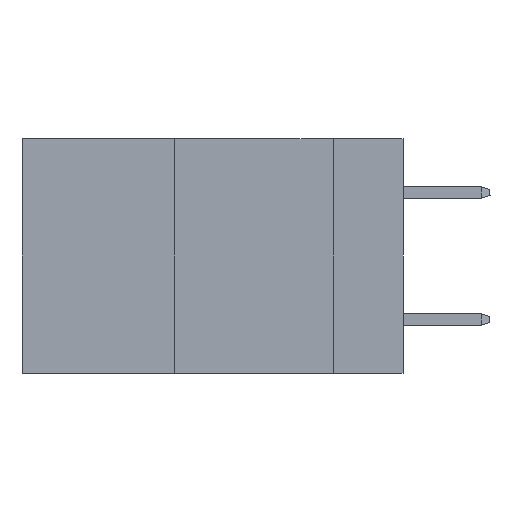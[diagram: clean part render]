
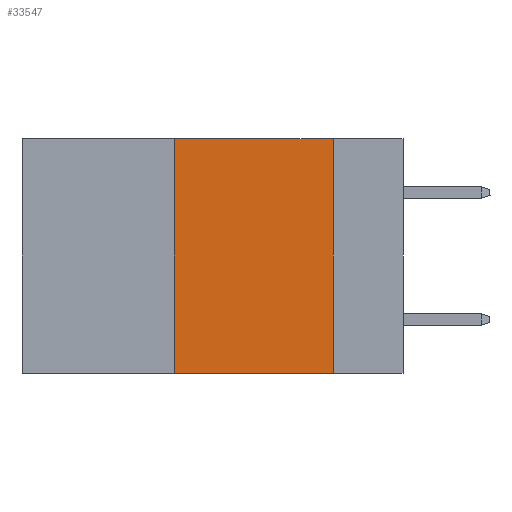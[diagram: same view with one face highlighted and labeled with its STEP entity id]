
A CAD part, left-side view. The second image highlights one B-rep face of the part: STEP entity #33547.
In plain terms, the highlighted planar face has unit normal (-1, 0, 0).
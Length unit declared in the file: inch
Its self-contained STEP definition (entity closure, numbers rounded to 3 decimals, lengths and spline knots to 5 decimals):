
#686 = VECTOR ( 'NONE', #26114, 39.37008 ) ;
#1525 = VERTEX_POINT ( 'NONE', #5872 ) ;
#2205 = EDGE_CURVE ( 'NONE', #9310, #1525, #44298, .T. ) ;
#3482 = DIRECTION ( 'NONE',  ( 0., -1., 0. ) ) ;
#5020 = ORIENTED_EDGE ( 'NONE', *, *, #42511, .F. ) ;
#5127 = EDGE_LOOP ( 'NONE', ( #23720, #5020, #41222, #33146 ) ) ;
#5872 = CARTESIAN_POINT ( 'NONE',  ( 0., 0.11, -0.37 ) ) ;
#6529 = VERTEX_POINT ( 'NONE', #11088 ) ;
#9310 = VERTEX_POINT ( 'NONE', #23360 ) ;
#9339 = LINE ( 'NONE', #17311, #20609 ) ;
#10568 = VERTEX_POINT ( 'NONE', #29339 ) ;
#11088 = CARTESIAN_POINT ( 'NONE',  ( 0., 0.36, 0. ) ) ;
#13699 = VECTOR ( 'NONE', #40795, 39.37008 ) ;
#15322 = EDGE_CURVE ( 'NONE', #10568, #6529, #9339, .T. ) ;
#17311 = CARTESIAN_POINT ( 'NONE',  ( 0., 0.36, 0. ) ) ;
#19581 = AXIS2_PLACEMENT_3D ( 'NONE', #23146, #37807, #26535 ) ;
#20609 = VECTOR ( 'NONE', #24756, 39.37008 ) ;
#22548 = CARTESIAN_POINT ( 'NONE',  ( 0., 0.6, -0.37 ) ) ;
#22710 = CARTESIAN_POINT ( 'NONE',  ( 0., 0.11, 0. ) ) ;
#23146 = CARTESIAN_POINT ( 'NONE',  ( 0., 0.6, 0. ) ) ;
#23360 = CARTESIAN_POINT ( 'NONE',  ( 0., 0.11, 0. ) ) ;
#23720 = ORIENTED_EDGE ( 'NONE', *, *, #2205, .F. ) ;
#24756 = DIRECTION ( 'NONE',  ( 0., 0., 1. ) ) ;
#26114 = DIRECTION ( 'NONE',  ( 0., 0., -1. ) ) ;
#26195 = LINE ( 'NONE', #22548, #13699 ) ;
#26535 = DIRECTION ( 'NONE',  ( 0., 0., -1. ) ) ;
#27465 = EDGE_CURVE ( 'NONE', #10568, #1525, #26195, .T. ) ;
#28939 = LINE ( 'NONE', #32077, #34560 ) ;
#29339 = CARTESIAN_POINT ( 'NONE',  ( 0., 0.36, -0.37 ) ) ;
#32077 = CARTESIAN_POINT ( 'NONE',  ( 0., 0.6, 0. ) ) ;
#33146 = ORIENTED_EDGE ( 'NONE', *, *, #27465, .T. ) ;
#33547 = ADVANCED_FACE ( 'NONE', ( #44727 ), #45427, .F. ) ;
#34560 = VECTOR ( 'NONE', #3482, 39.37008 ) ;
#37807 = DIRECTION ( 'NONE',  ( 1., 0., 0. ) ) ;
#40795 = DIRECTION ( 'NONE',  ( 0., -1., 0. ) ) ;
#41222 = ORIENTED_EDGE ( 'NONE', *, *, #15322, .F. ) ;
#42511 = EDGE_CURVE ( 'NONE', #6529, #9310, #28939, .T. ) ;
#44298 = LINE ( 'NONE', #22710, #686 ) ;
#44727 = FACE_OUTER_BOUND ( 'NONE', #5127, .T. ) ;
#45427 = PLANE ( 'NONE',  #19581 ) ;
